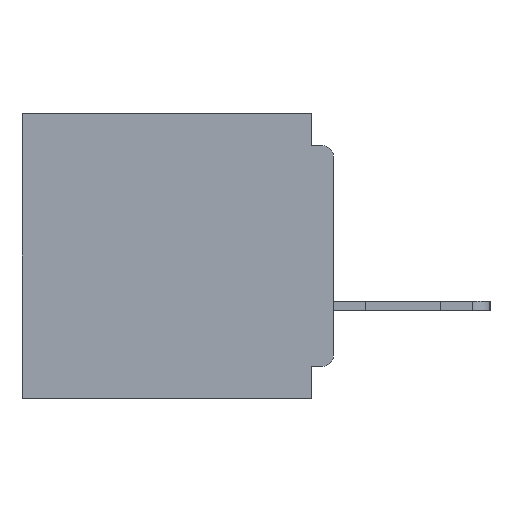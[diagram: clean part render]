
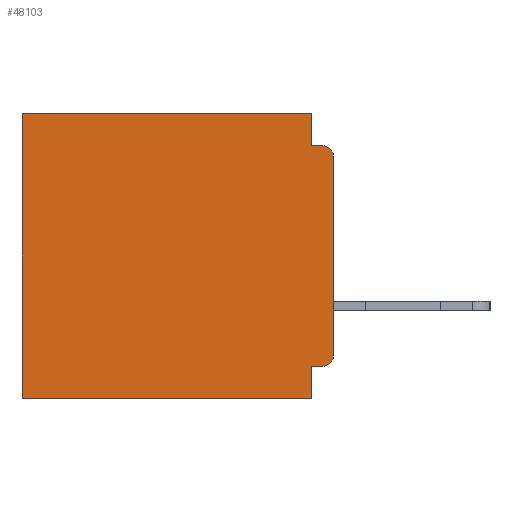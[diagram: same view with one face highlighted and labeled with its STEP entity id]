
A CAD part, left-side view. The second image highlights one B-rep face of the part: STEP entity #48103.
In plain terms, the highlighted planar face has unit normal (-1, 0, 0).
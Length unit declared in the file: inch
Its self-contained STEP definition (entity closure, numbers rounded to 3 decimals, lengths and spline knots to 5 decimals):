
#703 = DIRECTION ( 'NONE',  ( 0., 1., 0. ) ) ;
#1102 = CARTESIAN_POINT ( 'NONE',  ( 0.3, 0., -0.4 ) ) ;
#1790 = ORIENTED_EDGE ( 'NONE', *, *, #3149, .F. ) ;
#1987 = ORIENTED_EDGE ( 'NONE', *, *, #20795, .F. ) ;
#2207 = CARTESIAN_POINT ( 'NONE',  ( 0.3, 0.015, -0.34 ) ) ;
#2428 = CARTESIAN_POINT ( 'NONE',  ( 0.3, 0.031, 0. ) ) ;
#2705 = CARTESIAN_POINT ( 'NONE',  ( 0.3, 0.437, -0.4 ) ) ;
#2901 = CARTESIAN_POINT ( 'NONE',  ( 0.3, 0.015, -0.06 ) ) ;
#3149 = EDGE_CURVE ( 'NONE', #46304, #39552, #33749, .T. ) ;
#3320 = VECTOR ( 'NONE', #29306, 39.37008 ) ;
#5124 = FACE_OUTER_BOUND ( 'NONE', #19964, .T. ) ;
#6211 = CARTESIAN_POINT ( 'NONE',  ( 0.3, 0., -0.355 ) ) ;
#6925 = DIRECTION ( 'NONE',  ( 0., 0., -1. ) ) ;
#7601 = DIRECTION ( 'NONE',  ( 0., 0., -1. ) ) ;
#7856 = VERTEX_POINT ( 'NONE', #2428 ) ;
#8564 = ORIENTED_EDGE ( 'NONE', *, *, #23286, .F. ) ;
#9053 = EDGE_CURVE ( 'NONE', #26851, #39552, #29945, .T. ) ;
#9906 = CARTESIAN_POINT ( 'NONE',  ( 0.3, 0., -0.045 ) ) ;
#10372 = VECTOR ( 'NONE', #703, 39.37008 ) ;
#10938 = DIRECTION ( 'NONE',  ( 0., 1., 0. ) ) ;
#11325 = CARTESIAN_POINT ( 'NONE',  ( 0.3, 0.437, 0. ) ) ;
#13325 = CARTESIAN_POINT ( 'NONE',  ( 0.3, 0., -0.4 ) ) ;
#14264 = EDGE_CURVE ( 'NONE', #33706, #56270, #36820, .T. ) ;
#15172 = AXIS2_PLACEMENT_3D ( 'NONE', #2207, #34954, #6925 ) ;
#15729 = CARTESIAN_POINT ( 'NONE',  ( 0.3, 0., -0.06 ) ) ;
#18060 = DIRECTION ( 'NONE',  ( 0., 0., -1. ) ) ;
#19353 = DIRECTION ( 'NONE',  ( 0., -1., 0. ) ) ;
#19964 = EDGE_LOOP ( 'NONE', ( #1987, #45306, #59855, #48124, #20480, #36973, #1790, #24631, #8564, #30882 ) ) ;
#20149 = LINE ( 'NONE', #42770, #32527 ) ;
#20480 = ORIENTED_EDGE ( 'NONE', *, *, #35315, .T. ) ;
#20783 = CARTESIAN_POINT ( 'NONE',  ( 0.3, 0.437, -0.4 ) ) ;
#20795 = EDGE_CURVE ( 'NONE', #33706, #55380, #41119, .T. ) ;
#20825 = LINE ( 'NONE', #54747, #44257 ) ;
#21019 = CARTESIAN_POINT ( 'NONE',  ( 0.3, 0.031, -0.355 ) ) ;
#21059 = LINE ( 'NONE', #6211, #44477 ) ;
#22757 = CARTESIAN_POINT ( 'NONE',  ( 0.3, 0., -0.34 ) ) ;
#23286 = EDGE_CURVE ( 'NONE', #26252, #49111, #21059, .T. ) ;
#24631 = ORIENTED_EDGE ( 'NONE', *, *, #45315, .F. ) ;
#24737 = VERTEX_POINT ( 'NONE', #59599 ) ;
#25958 = EDGE_CURVE ( 'NONE', #7856, #24737, #20825, .T. ) ;
#26252 = VERTEX_POINT ( 'NONE', #57162 ) ;
#26573 = VECTOR ( 'NONE', #19353, 39.37008 ) ;
#26672 = EDGE_CURVE ( 'NONE', #24737, #56270, #38961, .T. ) ;
#26851 = VERTEX_POINT ( 'NONE', #11325 ) ;
#27267 = PLANE ( 'NONE',  #31431 ) ;
#27318 = CIRCLE ( 'NONE', #15172, 0.015 ) ;
#29306 = DIRECTION ( 'NONE',  ( 0., 0., -1. ) ) ;
#29391 = DIRECTION ( 'NONE',  ( 0., 0., -1. ) ) ;
#29945 = LINE ( 'NONE', #2705, #54793 ) ;
#30783 = DIRECTION ( 'NONE',  ( 0., 0., -1. ) ) ;
#30882 = ORIENTED_EDGE ( 'NONE', *, *, #55739, .T. ) ;
#31431 = AXIS2_PLACEMENT_3D ( 'NONE', #13325, #46105, #18060 ) ;
#32527 = VECTOR ( 'NONE', #47522, 39.37008 ) ;
#33706 = VERTEX_POINT ( 'NONE', #15729 ) ;
#33749 = LINE ( 'NONE', #34625, #10372 ) ;
#33785 = CARTESIAN_POINT ( 'NONE',  ( 0.3, 0.031, -0.4 ) ) ;
#34625 = CARTESIAN_POINT ( 'NONE',  ( 0.3, 0., -0.4 ) ) ;
#34954 = DIRECTION ( 'NONE',  ( -1., 0., 0. ) ) ;
#35315 = EDGE_CURVE ( 'NONE', #7856, #26851, #20149, .T. ) ;
#35652 = DIRECTION ( 'NONE',  ( -1., 0., 0. ) ) ;
#36820 = CIRCLE ( 'NONE', #40366, 0.015 ) ;
#36973 = ORIENTED_EDGE ( 'NONE', *, *, #9053, .T. ) ;
#38961 = LINE ( 'NONE', #9906, #26573 ) ;
#39552 = VERTEX_POINT ( 'NONE', #20783 ) ;
#40366 = AXIS2_PLACEMENT_3D ( 'NONE', #2901, #35652, #7601 ) ;
#40663 = LINE ( 'NONE', #33785, #3320 ) ;
#41119 = LINE ( 'NONE', #1102, #52080 ) ;
#42770 = CARTESIAN_POINT ( 'NONE',  ( 0.3, 0., 0. ) ) ;
#44257 = VECTOR ( 'NONE', #59459, 39.37008 ) ;
#44477 = VECTOR ( 'NONE', #10938, 39.37008 ) ;
#45306 = ORIENTED_EDGE ( 'NONE', *, *, #14264, .T. ) ;
#45315 = EDGE_CURVE ( 'NONE', #49111, #46304, #40663, .T. ) ;
#46105 = DIRECTION ( 'NONE',  ( 1., 0., 0. ) ) ;
#46304 = VERTEX_POINT ( 'NONE', #55984 ) ;
#47522 = DIRECTION ( 'NONE',  ( 0., 1., 0. ) ) ;
#48103 = ADVANCED_FACE ( 'NONE', ( #5124 ), #27267, .F. ) ;
#48124 = ORIENTED_EDGE ( 'NONE', *, *, #25958, .F. ) ;
#49111 = VERTEX_POINT ( 'NONE', #21019 ) ;
#52080 = VECTOR ( 'NONE', #29391, 39.37008 ) ;
#52884 = CARTESIAN_POINT ( 'NONE',  ( 0.3, 0.015, -0.045 ) ) ;
#54747 = CARTESIAN_POINT ( 'NONE',  ( 0.3, 0.031, 0. ) ) ;
#54793 = VECTOR ( 'NONE', #30783, 39.37008 ) ;
#55380 = VERTEX_POINT ( 'NONE', #22757 ) ;
#55739 = EDGE_CURVE ( 'NONE', #26252, #55380, #27318, .T. ) ;
#55984 = CARTESIAN_POINT ( 'NONE',  ( 0.3, 0.031, -0.4 ) ) ;
#56270 = VERTEX_POINT ( 'NONE', #52884 ) ;
#57162 = CARTESIAN_POINT ( 'NONE',  ( 0.3, 0.015, -0.355 ) ) ;
#59459 = DIRECTION ( 'NONE',  ( 0., 0., -1. ) ) ;
#59599 = CARTESIAN_POINT ( 'NONE',  ( 0.3, 0.031, -0.045 ) ) ;
#59855 = ORIENTED_EDGE ( 'NONE', *, *, #26672, .F. ) ;
